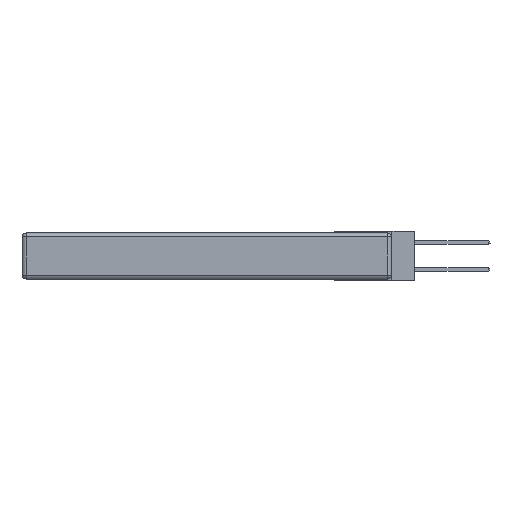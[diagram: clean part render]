
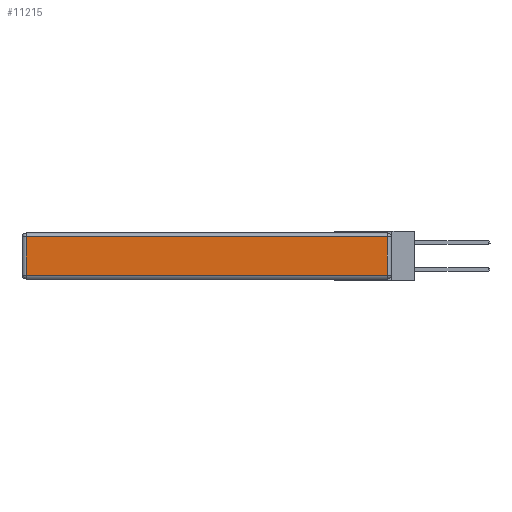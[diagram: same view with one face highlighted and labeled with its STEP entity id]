
A CAD part, left-side view. The second image highlights one B-rep face of the part: STEP entity #11215.
In plain terms, the highlighted planar face has unit normal (-1, 0, 0).
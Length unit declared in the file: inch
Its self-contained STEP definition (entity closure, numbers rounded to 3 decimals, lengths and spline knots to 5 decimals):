
#629 = ORIENTED_EDGE ( 'NONE', *, *, #15674, .T. ) ;
#1145 = EDGE_CURVE ( 'NONE', #15486, #20660, #21958, .T. ) ;
#1890 = CARTESIAN_POINT ( 'NONE',  ( 0., 0.03, -0.03 ) ) ;
#2684 = VECTOR ( 'NONE', #22105, 39.37008 ) ;
#2738 = CARTESIAN_POINT ( 'NONE',  ( 0., 2.72, -0.343 ) ) ;
#5389 = AXIS2_PLACEMENT_3D ( 'NONE', #17543, #9617, #9804 ) ;
#5525 = ORIENTED_EDGE ( 'NONE', *, *, #18938, .T. ) ;
#6990 = DIRECTION ( 'NONE',  ( 0., 1., 0. ) ) ;
#7217 = CARTESIAN_POINT ( 'NONE',  ( 0., 0.03, -0.343 ) ) ;
#7625 = FACE_OUTER_BOUND ( 'NONE', #12494, .T. ) ;
#9444 = VECTOR ( 'NONE', #22644, 39.37008 ) ;
#9469 = VECTOR ( 'NONE', #6990, 39.37008 ) ;
#9617 = DIRECTION ( 'NONE',  ( -1., 0., 0. ) ) ;
#9804 = DIRECTION ( 'NONE',  ( 0., 0., 1. ) ) ;
#11126 = LINE ( 'NONE', #15031, #2684 ) ;
#11215 = ADVANCED_FACE ( 'NONE', ( #7625 ), #23648, .T. ) ;
#11466 = EDGE_CURVE ( 'NONE', #17124, #15486, #14170, .T. ) ;
#12013 = CARTESIAN_POINT ( 'NONE',  ( 0., 0.03, -0.313 ) ) ;
#12494 = EDGE_LOOP ( 'NONE', ( #629, #5525, #18389, #24131 ) ) ;
#14170 = LINE ( 'NONE', #16913, #9469 ) ;
#14424 = VERTEX_POINT ( 'NONE', #12013 ) ;
#15031 = CARTESIAN_POINT ( 'NONE',  ( 0., 0., -0.313 ) ) ;
#15486 = VERTEX_POINT ( 'NONE', #20638 ) ;
#15674 = EDGE_CURVE ( 'NONE', #20660, #14424, #11126, .T. ) ;
#16913 = CARTESIAN_POINT ( 'NONE',  ( 0., 2.75, -0.03 ) ) ;
#17124 = VERTEX_POINT ( 'NONE', #1890 ) ;
#17543 = CARTESIAN_POINT ( 'NONE',  ( 0., 0., -0.343 ) ) ;
#18389 = ORIENTED_EDGE ( 'NONE', *, *, #11466, .T. ) ;
#18938 = EDGE_CURVE ( 'NONE', #14424, #17124, #20536, .T. ) ;
#20536 = LINE ( 'NONE', #7217, #25501 ) ;
#20638 = CARTESIAN_POINT ( 'NONE',  ( 0., 2.72, -0.03 ) ) ;
#20660 = VERTEX_POINT ( 'NONE', #24381 ) ;
#21256 = DIRECTION ( 'NONE',  ( 0., 0., 1. ) ) ;
#21958 = LINE ( 'NONE', #2738, #9444 ) ;
#22105 = DIRECTION ( 'NONE',  ( 0., -1., 0. ) ) ;
#22644 = DIRECTION ( 'NONE',  ( 0., 0., -1. ) ) ;
#23648 = PLANE ( 'NONE',  #5389 ) ;
#24131 = ORIENTED_EDGE ( 'NONE', *, *, #1145, .T. ) ;
#24381 = CARTESIAN_POINT ( 'NONE',  ( 0., 2.72, -0.313 ) ) ;
#25501 = VECTOR ( 'NONE', #21256, 39.37008 ) ;
